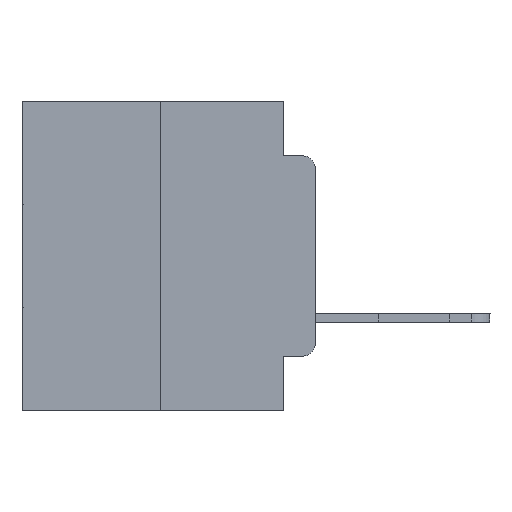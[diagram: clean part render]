
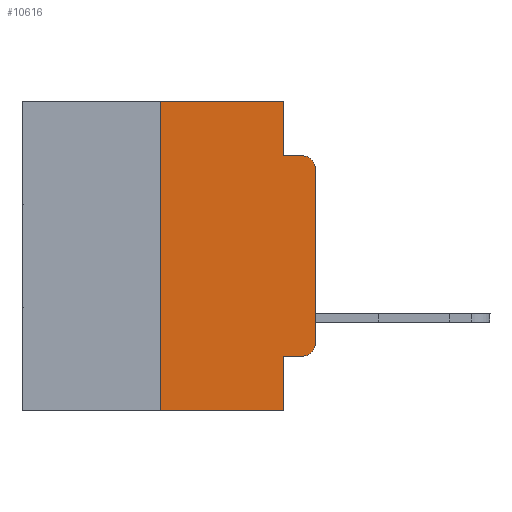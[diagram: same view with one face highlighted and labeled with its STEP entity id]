
A CAD part, left-side view. The second image highlights one B-rep face of the part: STEP entity #10616.
In plain terms, the highlighted planar face has unit normal (-1, 0, 0).
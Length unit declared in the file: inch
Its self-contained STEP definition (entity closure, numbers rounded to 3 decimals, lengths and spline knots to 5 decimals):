
#544 = ORIENTED_EDGE ( 'NONE', *, *, #20680, .F. ) ;
#1223 = VERTEX_POINT ( 'NONE', #21002 ) ;
#1438 = DIRECTION ( 'NONE',  ( 0., 0., -1. ) ) ;
#1542 = DIRECTION ( 'NONE',  ( 0., -1., 0. ) ) ;
#1710 = AXIS2_PLACEMENT_3D ( 'NONE', #20423, #14766, #17900 ) ;
#2052 = ORIENTED_EDGE ( 'NONE', *, *, #13484, .T. ) ;
#2452 = DIRECTION ( 'NONE',  ( 0., -1., 0. ) ) ;
#3217 = VERTEX_POINT ( 'NONE', #4767 ) ;
#3343 = CARTESIAN_POINT ( 'NONE',  ( 0., 0.051, 0. ) ) ;
#4250 = DIRECTION ( 'NONE',  ( 0., 0., 1. ) ) ;
#4453 = LINE ( 'NONE', #15623, #13278 ) ;
#4767 = CARTESIAN_POINT ( 'NONE',  ( 0., 0.051, -0.4115 ) ) ;
#4908 = CARTESIAN_POINT ( 'NONE',  ( 0., 0., 0. ) ) ;
#5033 = CARTESIAN_POINT ( 'NONE',  ( 0., 0.25, 0. ) ) ;
#5394 = VECTOR ( 'NONE', #1542, 39.37008 ) ;
#5404 = PLANE ( 'NONE',  #25814 ) ;
#5439 = DIRECTION ( 'NONE',  ( 0., 0., -1. ) ) ;
#5462 = VERTEX_POINT ( 'NONE', #5033 ) ;
#5832 = CARTESIAN_POINT ( 'NONE',  ( 0., 0.051, 0. ) ) ;
#6371 = VERTEX_POINT ( 'NONE', #7678 ) ;
#7229 = CARTESIAN_POINT ( 'NONE',  ( 0., 0.02, -0.3915 ) ) ;
#7400 = DIRECTION ( 'NONE',  ( 0., -1., 0. ) ) ;
#7508 = DIRECTION ( 'NONE',  ( -1., 0., 0. ) ) ;
#7678 = CARTESIAN_POINT ( 'NONE',  ( 0., 0., -0.3915 ) ) ;
#8104 = VECTOR ( 'NONE', #5439, 39.37008 ) ;
#9188 = ORIENTED_EDGE ( 'NONE', *, *, #25353, .T. ) ;
#9257 = AXIS2_PLACEMENT_3D ( 'NONE', #7229, #7508, #24821 ) ;
#9446 = ORIENTED_EDGE ( 'NONE', *, *, #20175, .F. ) ;
#9784 = ORIENTED_EDGE ( 'NONE', *, *, #18749, .F. ) ;
#10018 = VECTOR ( 'NONE', #23109, 39.37008 ) ;
#10616 = ADVANCED_FACE ( 'NONE', ( #15331 ), #5404, .F. ) ;
#10712 = CIRCLE ( 'NONE', #1710, 0.02 ) ;
#11254 = EDGE_CURVE ( 'NONE', #3217, #13526, #23159, .T. ) ;
#11523 = CARTESIAN_POINT ( 'NONE',  ( 0., 0.25, 0. ) ) ;
#12262 = CARTESIAN_POINT ( 'NONE',  ( 0., 0.473, 0. ) ) ;
#12652 = VECTOR ( 'NONE', #1438, 39.37008 ) ;
#12918 = CARTESIAN_POINT ( 'NONE',  ( 0., 0.25, -0.5 ) ) ;
#13260 = LINE ( 'NONE', #4908, #16000 ) ;
#13278 = VECTOR ( 'NONE', #2452, 39.37008 ) ;
#13484 = EDGE_CURVE ( 'NONE', #25348, #15240, #10712, .T. ) ;
#13526 = VERTEX_POINT ( 'NONE', #19053 ) ;
#13893 = LINE ( 'NONE', #3343, #8104 ) ;
#13896 = CARTESIAN_POINT ( 'NONE',  ( 0., 0.051, -0.5 ) ) ;
#14766 = DIRECTION ( 'NONE',  ( -1., 0., 0. ) ) ;
#14780 = LINE ( 'NONE', #16499, #10018 ) ;
#15240 = VERTEX_POINT ( 'NONE', #20201 ) ;
#15331 = FACE_OUTER_BOUND ( 'NONE', #25877, .T. ) ;
#15623 = CARTESIAN_POINT ( 'NONE',  ( 0., 0.473, -0.5 ) ) ;
#15650 = EDGE_CURVE ( 'NONE', #6371, #25348, #13260, .T. ) ;
#15801 = ORIENTED_EDGE ( 'NONE', *, *, #17340, .T. ) ;
#16000 = VECTOR ( 'NONE', #4250, 39.37008 ) ;
#16396 = EDGE_CURVE ( 'NONE', #23936, #1223, #13893, .T. ) ;
#16499 = CARTESIAN_POINT ( 'NONE',  ( 0., 0.473, 0. ) ) ;
#17340 = EDGE_CURVE ( 'NONE', #13526, #6371, #20346, .T. ) ;
#17900 = DIRECTION ( 'NONE',  ( 0., 0., -1. ) ) ;
#17910 = ORIENTED_EDGE ( 'NONE', *, *, #15650, .T. ) ;
#18098 = CARTESIAN_POINT ( 'NONE',  ( 0., 0., -0.1085 ) ) ;
#18749 = EDGE_CURVE ( 'NONE', #5462, #23936, #14780, .T. ) ;
#19053 = CARTESIAN_POINT ( 'NONE',  ( 0., 0.02, -0.4115 ) ) ;
#19589 = VECTOR ( 'NONE', #7400, 39.37008 ) ;
#19821 = VERTEX_POINT ( 'NONE', #12918 ) ;
#20175 = EDGE_CURVE ( 'NONE', #3217, #25621, #22902, .T. ) ;
#20201 = CARTESIAN_POINT ( 'NONE',  ( 0., 0.02, -0.0885 ) ) ;
#20346 = CIRCLE ( 'NONE', #9257, 0.02 ) ;
#20423 = CARTESIAN_POINT ( 'NONE',  ( 0., 0.02, -0.1085 ) ) ;
#20680 = EDGE_CURVE ( 'NONE', #19821, #5462, #28038, .T. ) ;
#20772 = ORIENTED_EDGE ( 'NONE', *, *, #16396, .F. ) ;
#21002 = CARTESIAN_POINT ( 'NONE',  ( 0., 0.051, -0.0885 ) ) ;
#22491 = EDGE_CURVE ( 'NONE', #1223, #15240, #23020, .T. ) ;
#22522 = ORIENTED_EDGE ( 'NONE', *, *, #22491, .F. ) ;
#22875 = VECTOR ( 'NONE', #24537, 39.37008 ) ;
#22902 = LINE ( 'NONE', #5832, #12652 ) ;
#23020 = LINE ( 'NONE', #25098, #19589 ) ;
#23109 = DIRECTION ( 'NONE',  ( 0., -1., 0. ) ) ;
#23159 = LINE ( 'NONE', #25156, #5394 ) ;
#23265 = DIRECTION ( 'NONE',  ( 1., 0., 0. ) ) ;
#23936 = VERTEX_POINT ( 'NONE', #27918 ) ;
#24537 = DIRECTION ( 'NONE',  ( 0., 0., 1. ) ) ;
#24799 = ORIENTED_EDGE ( 'NONE', *, *, #11254, .T. ) ;
#24821 = DIRECTION ( 'NONE',  ( 0., 0., -1. ) ) ;
#25098 = CARTESIAN_POINT ( 'NONE',  ( 0., 0.051, -0.0885 ) ) ;
#25156 = CARTESIAN_POINT ( 'NONE',  ( 0., 0.051, -0.4115 ) ) ;
#25348 = VERTEX_POINT ( 'NONE', #18098 ) ;
#25353 = EDGE_CURVE ( 'NONE', #19821, #25621, #4453, .T. ) ;
#25621 = VERTEX_POINT ( 'NONE', #13896 ) ;
#25814 = AXIS2_PLACEMENT_3D ( 'NONE', #12262, #23265, #27501 ) ;
#25877 = EDGE_LOOP ( 'NONE', ( #17910, #2052, #22522, #20772, #9784, #544, #9188, #9446, #24799, #15801 ) ) ;
#27501 = DIRECTION ( 'NONE',  ( 0., 0., -1. ) ) ;
#27918 = CARTESIAN_POINT ( 'NONE',  ( 0., 0.051, 0. ) ) ;
#28038 = LINE ( 'NONE', #11523, #22875 ) ;
